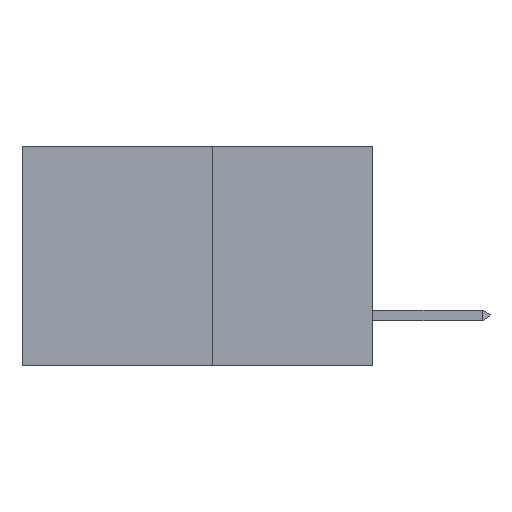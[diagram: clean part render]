
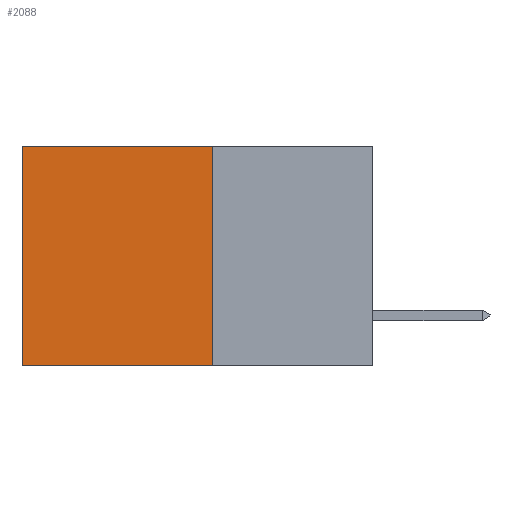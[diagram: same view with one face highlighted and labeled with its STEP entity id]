
A CAD part, left-side view. The second image highlights one B-rep face of the part: STEP entity #2088.
In plain terms, the highlighted planar face has unit normal (-1, 0, 0).
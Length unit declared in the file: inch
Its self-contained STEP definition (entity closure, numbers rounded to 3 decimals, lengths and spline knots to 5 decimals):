
#304 = VERTEX_POINT ( 'NONE', #2555 ) ;
#414 = FACE_OUTER_BOUND ( 'NONE', #4819, .T. ) ;
#500 = EDGE_CURVE ( 'NONE', #5118, #3130, #745, .T. ) ;
#745 = LINE ( 'NONE', #9131, #2791 ) ;
#1188 = EDGE_CURVE ( 'NONE', #7991, #3130, #6443, .T. ) ;
#1411 = DIRECTION ( 'NONE',  ( 0., 1., 0. ) ) ;
#1895 = CARTESIAN_POINT ( 'NONE',  ( 0.277, 0.27, -0.37 ) ) ;
#1965 = CARTESIAN_POINT ( 'NONE',  ( 0.277, 0.27, -0.37 ) ) ;
#1995 = CARTESIAN_POINT ( 'NONE',  ( 0.277, 0.59, -0.37 ) ) ;
#2088 = ADVANCED_FACE ( 'NONE', ( #414 ), #9254, .F. ) ;
#2555 = CARTESIAN_POINT ( 'NONE',  ( 0.277, 0.27, 0. ) ) ;
#2593 = ORIENTED_EDGE ( 'NONE', *, *, #500, .T. ) ;
#2646 = VECTOR ( 'NONE', #1411, 39.37008 ) ;
#2664 = ORIENTED_EDGE ( 'NONE', *, *, #5231, .F. ) ;
#2791 = VECTOR ( 'NONE', #5461, 39.37008 ) ;
#2884 = ORIENTED_EDGE ( 'NONE', *, *, #3465, .T. ) ;
#2945 = VECTOR ( 'NONE', #6261, 39.37008 ) ;
#3084 = DIRECTION ( 'NONE',  ( 0., 0., -1. ) ) ;
#3130 = VERTEX_POINT ( 'NONE', #1995 ) ;
#3241 = DIRECTION ( 'NONE',  ( 0., 0., -1. ) ) ;
#3465 = EDGE_CURVE ( 'NONE', #304, #5118, #8370, .T. ) ;
#3607 = ORIENTED_EDGE ( 'NONE', *, *, #1188, .F. ) ;
#3967 = CARTESIAN_POINT ( 'NONE',  ( 0.277, 0.27, -0.37 ) ) ;
#4427 = DIRECTION ( 'NONE',  ( 1., 0., 0. ) ) ;
#4682 = VECTOR ( 'NONE', #3084, 39.37008 ) ;
#4819 = EDGE_LOOP ( 'NONE', ( #2593, #3607, #2664, #2884 ) ) ;
#5118 = VERTEX_POINT ( 'NONE', #9086 ) ;
#5231 = EDGE_CURVE ( 'NONE', #304, #7991, #6502, .T. ) ;
#5361 = CARTESIAN_POINT ( 'NONE',  ( 0.277, 0.27, -0.37 ) ) ;
#5461 = DIRECTION ( 'NONE',  ( 0., 0., -1. ) ) ;
#6261 = DIRECTION ( 'NONE',  ( 0., 1., 0. ) ) ;
#6443 = LINE ( 'NONE', #3967, #2646 ) ;
#6502 = LINE ( 'NONE', #1965, #4682 ) ;
#7916 = AXIS2_PLACEMENT_3D ( 'NONE', #5361, #4427, #3241 ) ;
#7991 = VERTEX_POINT ( 'NONE', #1895 ) ;
#8370 = LINE ( 'NONE', #8675, #2945 ) ;
#8675 = CARTESIAN_POINT ( 'NONE',  ( 0.277, 0.27, 0. ) ) ;
#9086 = CARTESIAN_POINT ( 'NONE',  ( 0.277, 0.59, 0. ) ) ;
#9131 = CARTESIAN_POINT ( 'NONE',  ( 0.277, 0.59, -0.37 ) ) ;
#9254 = PLANE ( 'NONE',  #7916 ) ;
